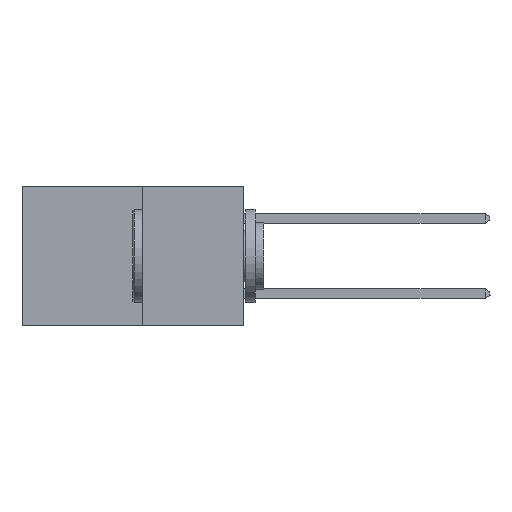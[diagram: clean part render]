
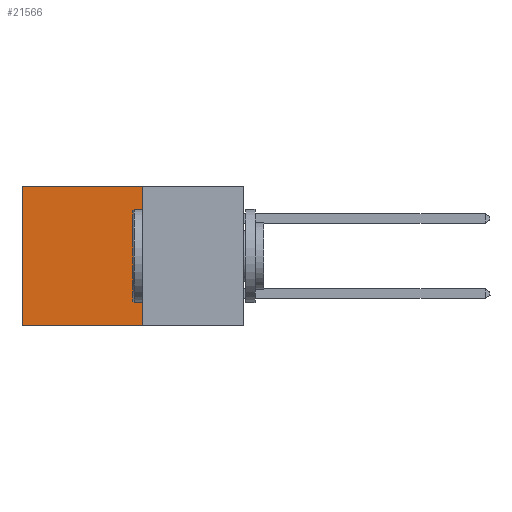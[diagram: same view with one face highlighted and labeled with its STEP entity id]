
A CAD part, left-side view. The second image highlights one B-rep face of the part: STEP entity #21566.
In plain terms, the highlighted planar face has unit normal (-1, 0, 0).
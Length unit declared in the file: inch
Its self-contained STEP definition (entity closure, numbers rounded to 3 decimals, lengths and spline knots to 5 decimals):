
#1085 = CARTESIAN_POINT ( 'NONE',  ( 0.277, 0.59, -0.37 ) ) ;
#1148 = FACE_OUTER_BOUND ( 'NONE', #10731, .T. ) ;
#1265 = ORIENTED_EDGE ( 'NONE', *, *, #10375, .T. ) ;
#3305 = AXIS2_PLACEMENT_3D ( 'NONE', #7821, #22370, #9949 ) ;
#4375 = LINE ( 'NONE', #15070, #14896 ) ;
#4565 = ORIENTED_EDGE ( 'NONE', *, *, #26073, .F. ) ;
#5141 = ORIENTED_EDGE ( 'NONE', *, *, #20757, .T. ) ;
#6092 = VERTEX_POINT ( 'NONE', #16032 ) ;
#7821 = CARTESIAN_POINT ( 'NONE',  ( 0.277, 0.27, -0.37 ) ) ;
#8471 = LINE ( 'NONE', #11424, #19530 ) ;
#9549 = CARTESIAN_POINT ( 'NONE',  ( 0.277, 0.27, 0. ) ) ;
#9641 = DIRECTION ( 'NONE',  ( 0., 1., 0. ) ) ;
#9949 = DIRECTION ( 'NONE',  ( 0., 0., -1. ) ) ;
#10242 = VERTEX_POINT ( 'NONE', #11491 ) ;
#10375 = EDGE_CURVE ( 'NONE', #10242, #16513, #25334, .T. ) ;
#10491 = LINE ( 'NONE', #1085, #26401 ) ;
#10731 = EDGE_LOOP ( 'NONE', ( #5141, #4565, #16299, #1265 ) ) ;
#10774 = CARTESIAN_POINT ( 'NONE',  ( 0.277, 0.59, 0. ) ) ;
#11424 = CARTESIAN_POINT ( 'NONE',  ( 0.277, 0.27, -0.37 ) ) ;
#11491 = CARTESIAN_POINT ( 'NONE',  ( 0.277, 0.27, 0. ) ) ;
#11742 = DIRECTION ( 'NONE',  ( 0., 0., -1. ) ) ;
#12979 = DIRECTION ( 'NONE',  ( 0., 1., 0. ) ) ;
#14896 = VECTOR ( 'NONE', #12979, 39.37008 ) ;
#15070 = CARTESIAN_POINT ( 'NONE',  ( 0.277, 0.27, -0.37 ) ) ;
#16032 = CARTESIAN_POINT ( 'NONE',  ( 0.277, 0.27, -0.37 ) ) ;
#16035 = EDGE_CURVE ( 'NONE', #10242, #6092, #8471, .T. ) ;
#16167 = PLANE ( 'NONE',  #3305 ) ;
#16299 = ORIENTED_EDGE ( 'NONE', *, *, #16035, .F. ) ;
#16513 = VERTEX_POINT ( 'NONE', #10774 ) ;
#19530 = VECTOR ( 'NONE', #23878, 39.37008 ) ;
#20453 = VECTOR ( 'NONE', #9641, 39.37008 ) ;
#20757 = EDGE_CURVE ( 'NONE', #16513, #25248, #10491, .T. ) ;
#21566 = ADVANCED_FACE ( 'NONE', ( #1148 ), #16167, .F. ) ;
#22370 = DIRECTION ( 'NONE',  ( 1., 0., 0. ) ) ;
#23878 = DIRECTION ( 'NONE',  ( 0., 0., -1. ) ) ;
#25248 = VERTEX_POINT ( 'NONE', #27053 ) ;
#25334 = LINE ( 'NONE', #9549, #20453 ) ;
#26073 = EDGE_CURVE ( 'NONE', #6092, #25248, #4375, .T. ) ;
#26401 = VECTOR ( 'NONE', #11742, 39.37008 ) ;
#27053 = CARTESIAN_POINT ( 'NONE',  ( 0.277, 0.59, -0.37 ) ) ;
